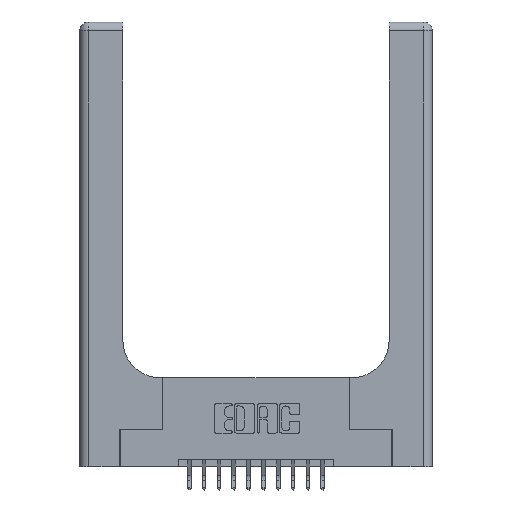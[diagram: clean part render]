
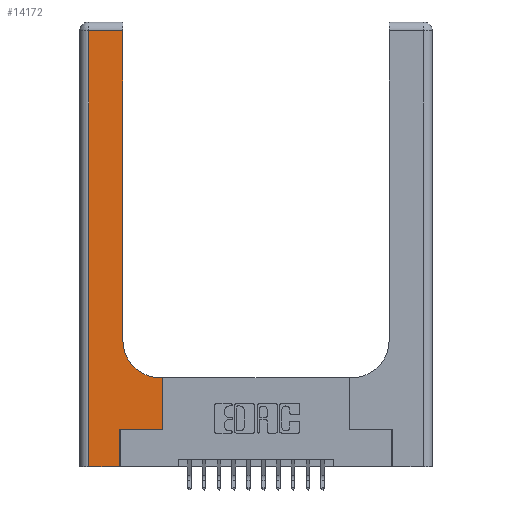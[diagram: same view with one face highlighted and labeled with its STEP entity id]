
A CAD part, top view. The second image highlights one B-rep face of the part: STEP entity #14172.
In plain terms, the highlighted planar face has unit normal (0, 0, 1).
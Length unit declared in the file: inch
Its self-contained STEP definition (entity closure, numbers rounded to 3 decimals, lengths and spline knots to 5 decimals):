
#193 = CARTESIAN_POINT ( 'NONE',  ( 0., 2.94, 0.37 ) ) ;
#245 = ORIENTED_EDGE ( 'NONE', *, *, #965, .T. ) ;
#352 = CARTESIAN_POINT ( 'NONE',  ( 0.5415, 0.6, 0.37 ) ) ;
#699 = ORIENTED_EDGE ( 'NONE', *, *, #14409, .T. ) ;
#868 = DIRECTION ( 'NONE',  ( -1., 0., 0. ) ) ;
#965 = EDGE_CURVE ( 'NONE', #5193, #3480, #3593, .T. ) ;
#1580 = VECTOR ( 'NONE', #5386, 39.37008 ) ;
#1618 = CARTESIAN_POINT ( 'NONE',  ( 0.269, 0., 0.37 ) ) ;
#1638 = PLANE ( 'NONE',  #5281 ) ;
#1864 = CARTESIAN_POINT ( 'NONE',  ( 0.2915, 0.85, 0.37 ) ) ;
#2006 = ORIENTED_EDGE ( 'NONE', *, *, #13964, .T. ) ;
#2144 = DIRECTION ( 'NONE',  ( 1., 0., 0. ) ) ;
#2387 = EDGE_LOOP ( 'NONE', ( #245, #14731, #699, #8397, #15566, #2006, #9257, #6073, #3329 ) ) ;
#2615 = LINE ( 'NONE', #11792, #17379 ) ;
#2639 = LINE ( 'NONE', #17089, #6677 ) ;
#3052 = DIRECTION ( 'NONE',  ( -1., 0., 0. ) ) ;
#3081 = EDGE_CURVE ( 'NONE', #11748, #9677, #8846, .T. ) ;
#3329 = ORIENTED_EDGE ( 'NONE', *, *, #11683, .T. ) ;
#3480 = VERTEX_POINT ( 'NONE', #12797 ) ;
#3593 = LINE ( 'NONE', #10845, #17079 ) ;
#3630 = CARTESIAN_POINT ( 'NONE',  ( 0.06, 0., 0.37 ) ) ;
#4023 = AXIS2_PLACEMENT_3D ( 'NONE', #4641, #14087, #5994 ) ;
#4032 = CIRCLE ( 'NONE', #4023, 0.25 ) ;
#4235 = EDGE_CURVE ( 'NONE', #12739, #7467, #2639, .T. ) ;
#4641 = CARTESIAN_POINT ( 'NONE',  ( 0.5415, 0.85, 0.37 ) ) ;
#5193 = VERTEX_POINT ( 'NONE', #1864 ) ;
#5281 = AXIS2_PLACEMENT_3D ( 'NONE', #9807, #11154, #3052 ) ;
#5386 = DIRECTION ( 'NONE',  ( 1., 0., 0. ) ) ;
#5591 = CARTESIAN_POINT ( 'NONE',  ( 0., 0., 0.37 ) ) ;
#5712 = LINE ( 'NONE', #1618, #12501 ) ;
#5994 = DIRECTION ( 'NONE',  ( 1., 0., 0. ) ) ;
#6073 = ORIENTED_EDGE ( 'NONE', *, *, #4235, .T. ) ;
#6677 = VECTOR ( 'NONE', #868, 39.37008 ) ;
#6960 = CARTESIAN_POINT ( 'NONE',  ( 0.06, 2.94, 0.37 ) ) ;
#7467 = VERTEX_POINT ( 'NONE', #352 ) ;
#7508 = CARTESIAN_POINT ( 'NONE',  ( 0.269, 0.25, 0.37 ) ) ;
#8246 = CARTESIAN_POINT ( 'NONE',  ( 0.5585, 0.25, 0.37 ) ) ;
#8294 = CARTESIAN_POINT ( 'NONE',  ( 0.269, 0.25, 0.37 ) ) ;
#8397 = ORIENTED_EDGE ( 'NONE', *, *, #3081, .T. ) ;
#8489 = VECTOR ( 'NONE', #12572, 39.37008 ) ;
#8741 = CARTESIAN_POINT ( 'NONE',  ( 0.5585, 0.6, 0.37 ) ) ;
#8846 = LINE ( 'NONE', #5591, #1580 ) ;
#9013 = LINE ( 'NONE', #7508, #15738 ) ;
#9099 = VERTEX_POINT ( 'NONE', #6960 ) ;
#9257 = ORIENTED_EDGE ( 'NONE', *, *, #16407, .T. ) ;
#9677 = VERTEX_POINT ( 'NONE', #12449 ) ;
#9807 = CARTESIAN_POINT ( 'NONE',  ( 0., 3., 0.37 ) ) ;
#10060 = FACE_OUTER_BOUND ( 'NONE', #2387, .T. ) ;
#10204 = VERTEX_POINT ( 'NONE', #8294 ) ;
#10673 = DIRECTION ( 'NONE',  ( 0., 1., 0. ) ) ;
#10845 = CARTESIAN_POINT ( 'NONE',  ( 0.2915, 3., 0.37 ) ) ;
#11154 = DIRECTION ( 'NONE',  ( 0., 0., -1. ) ) ;
#11195 = CARTESIAN_POINT ( 'NONE',  ( 0.5585, 0.25, 0.37 ) ) ;
#11415 = VERTEX_POINT ( 'NONE', #8246 ) ;
#11487 = VECTOR ( 'NONE', #15179, 39.37008 ) ;
#11575 = EDGE_CURVE ( 'NONE', #9677, #10204, #5712, .T. ) ;
#11683 = EDGE_CURVE ( 'NONE', #7467, #5193, #4032, .T. ) ;
#11748 = VERTEX_POINT ( 'NONE', #3630 ) ;
#11792 = CARTESIAN_POINT ( 'NONE',  ( 0.06, 3., 0.37 ) ) ;
#11915 = LINE ( 'NONE', #193, #11487 ) ;
#12449 = CARTESIAN_POINT ( 'NONE',  ( 0.269, 0., 0.37 ) ) ;
#12501 = VECTOR ( 'NONE', #12515, 39.37008 ) ;
#12515 = DIRECTION ( 'NONE',  ( 0., 1., 0. ) ) ;
#12572 = DIRECTION ( 'NONE',  ( 0., 1., 0. ) ) ;
#12739 = VERTEX_POINT ( 'NONE', #8741 ) ;
#12797 = CARTESIAN_POINT ( 'NONE',  ( 0.2915, 2.94, 0.37 ) ) ;
#13166 = DIRECTION ( 'NONE',  ( 0., -1., 0. ) ) ;
#13964 = EDGE_CURVE ( 'NONE', #10204, #11415, #9013, .T. ) ;
#14087 = DIRECTION ( 'NONE',  ( 0., 0., -1. ) ) ;
#14172 = ADVANCED_FACE ( 'NONE', ( #10060 ), #1638, .F. ) ;
#14409 = EDGE_CURVE ( 'NONE', #9099, #11748, #2615, .T. ) ;
#14731 = ORIENTED_EDGE ( 'NONE', *, *, #15294, .T. ) ;
#15179 = DIRECTION ( 'NONE',  ( -1., 0., 0. ) ) ;
#15294 = EDGE_CURVE ( 'NONE', #3480, #9099, #11915, .T. ) ;
#15566 = ORIENTED_EDGE ( 'NONE', *, *, #11575, .T. ) ;
#15661 = LINE ( 'NONE', #11195, #8489 ) ;
#15738 = VECTOR ( 'NONE', #2144, 39.37008 ) ;
#16407 = EDGE_CURVE ( 'NONE', #11415, #12739, #15661, .T. ) ;
#17079 = VECTOR ( 'NONE', #10673, 39.37008 ) ;
#17089 = CARTESIAN_POINT ( 'NONE',  ( 0.2915, 0.6, 0.37 ) ) ;
#17379 = VECTOR ( 'NONE', #13166, 39.37008 ) ;
